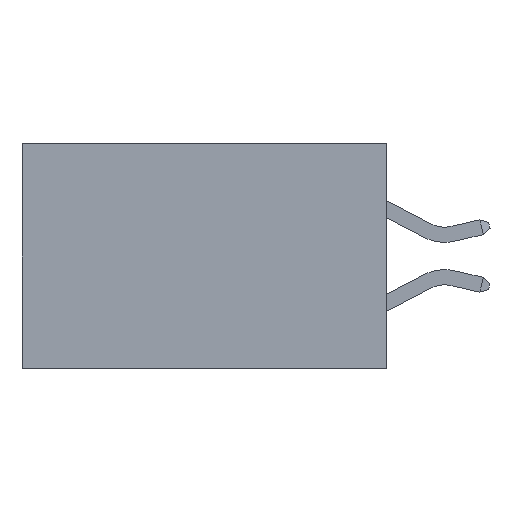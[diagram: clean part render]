
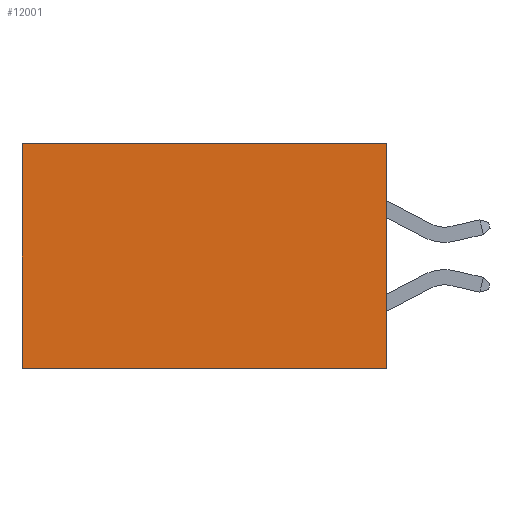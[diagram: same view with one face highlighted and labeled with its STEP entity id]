
A CAD part, left-side view. The second image highlights one B-rep face of the part: STEP entity #12001.
In plain terms, the highlighted planar face has unit normal (-1, 0, 0).
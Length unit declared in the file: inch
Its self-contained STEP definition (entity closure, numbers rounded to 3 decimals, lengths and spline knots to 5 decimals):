
#115 = LINE ( 'NONE', #14256, #10163 ) ;
#385 = VERTEX_POINT ( 'NONE', #10941 ) ;
#2058 = ORIENTED_EDGE ( 'NONE', *, *, #2995, .F. ) ;
#2322 = VERTEX_POINT ( 'NONE', #7729 ) ;
#2995 = EDGE_CURVE ( 'NONE', #2322, #385, #10826, .T. ) ;
#3656 = CARTESIAN_POINT ( 'NONE',  ( 0.2615, 0., 0. ) ) ;
#4020 = EDGE_CURVE ( 'NONE', #11261, #385, #115, .T. ) ;
#4066 = EDGE_CURVE ( 'NONE', #11421, #11261, #8630, .T. ) ;
#4145 = ORIENTED_EDGE ( 'NONE', *, *, #11129, .F. ) ;
#4985 = CARTESIAN_POINT ( 'NONE',  ( 0.2615, 0., -0.37 ) ) ;
#6942 = DIRECTION ( 'NONE',  ( 0., 0., -1. ) ) ;
#7729 = CARTESIAN_POINT ( 'NONE',  ( 0.2615, 0., -0.37 ) ) ;
#8630 = LINE ( 'NONE', #3656, #10659 ) ;
#9042 = VECTOR ( 'NONE', #10897, 39.37008 ) ;
#9240 = LINE ( 'NONE', #15088, #14473 ) ;
#10163 = VECTOR ( 'NONE', #14173, 39.37008 ) ;
#10297 = AXIS2_PLACEMENT_3D ( 'NONE', #14278, #10816, #12968 ) ;
#10659 = VECTOR ( 'NONE', #11797, 39.37008 ) ;
#10733 = PLANE ( 'NONE',  #10297 ) ;
#10816 = DIRECTION ( 'NONE',  ( 1., 0., 0. ) ) ;
#10826 = LINE ( 'NONE', #4985, #9042 ) ;
#10897 = DIRECTION ( 'NONE',  ( 0., 1., 0. ) ) ;
#10941 = CARTESIAN_POINT ( 'NONE',  ( 0.2615, 0.6, -0.37 ) ) ;
#11104 = CARTESIAN_POINT ( 'NONE',  ( 0.2615, 0.6, 0. ) ) ;
#11129 = EDGE_CURVE ( 'NONE', #11421, #2322, #9240, .T. ) ;
#11261 = VERTEX_POINT ( 'NONE', #11104 ) ;
#11421 = VERTEX_POINT ( 'NONE', #13994 ) ;
#11450 = EDGE_LOOP ( 'NONE', ( #11538, #2058, #4145, #14328 ) ) ;
#11538 = ORIENTED_EDGE ( 'NONE', *, *, #4020, .T. ) ;
#11797 = DIRECTION ( 'NONE',  ( 0., 1., 0. ) ) ;
#12001 = ADVANCED_FACE ( 'NONE', ( #14197 ), #10733, .F. ) ;
#12968 = DIRECTION ( 'NONE',  ( 0., 0., -1. ) ) ;
#13994 = CARTESIAN_POINT ( 'NONE',  ( 0.2615, 0., 0. ) ) ;
#14173 = DIRECTION ( 'NONE',  ( 0., 0., -1. ) ) ;
#14197 = FACE_OUTER_BOUND ( 'NONE', #11450, .T. ) ;
#14256 = CARTESIAN_POINT ( 'NONE',  ( 0.2615, 0.6, -0.37 ) ) ;
#14278 = CARTESIAN_POINT ( 'NONE',  ( 0.2615, 0., -0.37 ) ) ;
#14328 = ORIENTED_EDGE ( 'NONE', *, *, #4066, .T. ) ;
#14473 = VECTOR ( 'NONE', #6942, 39.37008 ) ;
#15088 = CARTESIAN_POINT ( 'NONE',  ( 0.2615, 0., -0.37 ) ) ;
